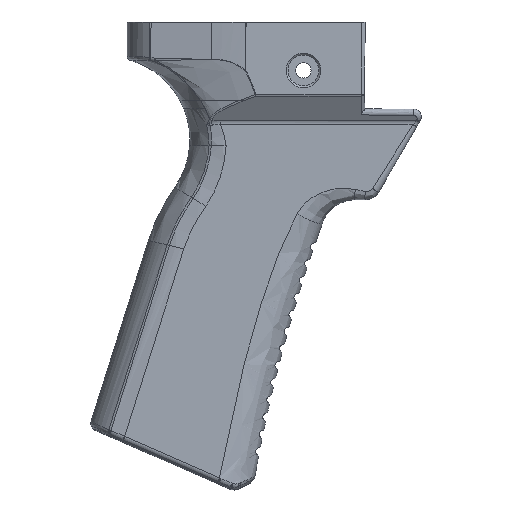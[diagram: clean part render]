
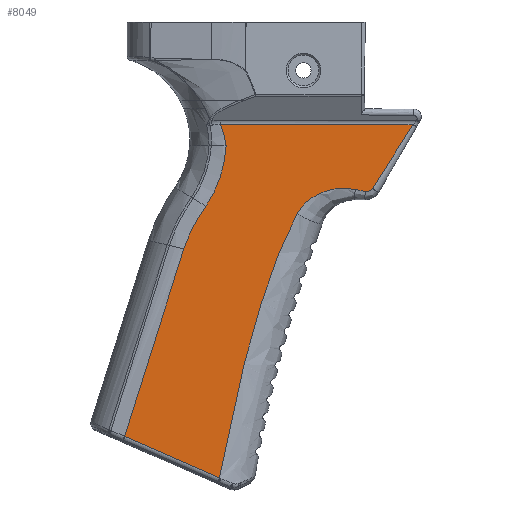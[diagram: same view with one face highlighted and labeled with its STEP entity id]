
A CAD part, front view. The second image highlights one B-rep face of the part: STEP entity #8049.
In plain terms, the highlighted planar face has unit normal (0, -1, 0).
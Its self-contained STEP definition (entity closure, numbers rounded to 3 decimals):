
#165=PLANE('',#8667);
#487=CIRCLE('',#8652,40.554);
#494=CIRCLE('',#8668,30.927);
#1096=FACE_OUTER_BOUND('',#1602,.T.);
#1602=EDGE_LOOP('',(#6779,#6780,#6781,#6782,#6783,#6784,#6785,#6786,#6787,
#6788,#6789,#6790,#6791,#6792));
#1988=LINE('',#18646,#2397);
#1993=LINE('',#19076,#2402);
#2001=LINE('',#19854,#2410);
#2397=VECTOR('',#9956,10.);
#2402=VECTOR('',#9979,10.);
#2410=VECTOR('',#10015,10.);
#2932=B_SPLINE_CURVE_WITH_KNOTS('',3,(#18666,#18667,#18668,#18669),
 .UNSPECIFIED.,.F.,.F.,(4,4),(0.,0.01),.UNSPECIFIED.);
#2937=B_SPLINE_CURVE_WITH_KNOTS('',3,(#18757,#18758,#18759,#18760),
 .UNSPECIFIED.,.F.,.F.,(4,4),(0.,0.007),.UNSPECIFIED.);
#2941=B_SPLINE_CURVE_WITH_KNOTS('',3,(#18888,#18889,#18890,#18891,#18892,
#18893,#18894,#18895,#18896),.UNSPECIFIED.,.F.,.F.,(4,1,1,1,1,1,4),(6.035,
6.926,7.817,9.599,11.381,13.163,
13.222),.UNSPECIFIED.);
#2953=B_SPLINE_CURVE_WITH_KNOTS('',3,(#19226,#19227,#19228,#19229,#19230,
#19231,#19232),.UNSPECIFIED.,.F.,.F.,(4,1,1,1,4),(4.224,5.,
5.518,5.776,5.862),.UNSPECIFIED.);
#2954=B_SPLINE_CURVE_WITH_KNOTS('',3,(#19233,#19234,#19235,#19236),
 .UNSPECIFIED.,.F.,.F.,(4,4),(5.862,6.035),
 .UNSPECIFIED.);
#2956=B_SPLINE_CURVE_WITH_KNOTS('',3,(#19274,#19275,#19276,#19277),
 .UNSPECIFIED.,.F.,.F.,(4,4),(3.956,4.224),
 .UNSPECIFIED.);
#2959=B_SPLINE_CURVE_WITH_KNOTS('',3,(#19326,#19327,#19328,#19329,#19330),
 .UNSPECIFIED.,.F.,.F.,(4,1,4),(3.743,3.835,3.956),
 .UNSPECIFIED.);
#2962=B_SPLINE_CURVE_WITH_KNOTS('',3,(#19380,#19381,#19382,#19383,#19384),
 .UNSPECIFIED.,.F.,.F.,(4,1,4),(1.774,2.899,3.743),
 .UNSPECIFIED.);
#2976=B_SPLINE_CURVE_WITH_KNOTS('',3,(#19856,#19857,#19858,#19859,#19860,
#19861,#19862),.UNSPECIFIED.,.F.,.F.,(4,3,4),(0.258,0.274,
0.412),.UNSPECIFIED.);
#3595=VERTEX_POINT('',#18643);
#3596=VERTEX_POINT('',#18645);
#3597=VERTEX_POINT('',#18664);
#3599=VERTEX_POINT('',#18708);
#3602=VERTEX_POINT('',#18880);
#3608=VERTEX_POINT('',#19011);
#3609=VERTEX_POINT('',#19019);
#3618=VERTEX_POINT('',#19217);
#3619=VERTEX_POINT('',#19225);
#3621=VERTEX_POINT('',#19266);
#3623=VERTEX_POINT('',#19318);
#3625=VERTEX_POINT('',#19372);
#3634=VERTEX_POINT('',#19853);
#3635=VERTEX_POINT('',#19855);
#4657=EDGE_CURVE('',#3595,#3596,#1988,.T.);
#4660=EDGE_CURVE('',#3596,#3597,#2932,.T.);
#4668=EDGE_CURVE('',#3597,#3599,#2937,.T.);
#4672=EDGE_CURVE('',#3602,#3595,#2941,.T.);
#4684=EDGE_CURVE('',#3608,#3609,#487,.T.);
#4687=EDGE_CURVE('',#3609,#3599,#1993,.T.);
#4703=EDGE_CURVE('',#3618,#3619,#2953,.T.);
#4704=EDGE_CURVE('',#3619,#3602,#2954,.T.);
#4706=EDGE_CURVE('',#3621,#3618,#2956,.T.);
#4709=EDGE_CURVE('',#3623,#3621,#2959,.T.);
#4712=EDGE_CURVE('',#3625,#3623,#2962,.T.);
#4728=EDGE_CURVE('',#3634,#3625,#2001,.T.);
#4729=EDGE_CURVE('',#3635,#3634,#2976,.T.);
#4730=EDGE_CURVE('',#3635,#3608,#494,.T.);
#6779=ORIENTED_EDGE('',*,*,#4703,.F.);
#6780=ORIENTED_EDGE('',*,*,#4706,.F.);
#6781=ORIENTED_EDGE('',*,*,#4709,.F.);
#6782=ORIENTED_EDGE('',*,*,#4712,.F.);
#6783=ORIENTED_EDGE('',*,*,#4728,.F.);
#6784=ORIENTED_EDGE('',*,*,#4729,.F.);
#6785=ORIENTED_EDGE('',*,*,#4730,.T.);
#6786=ORIENTED_EDGE('',*,*,#4684,.T.);
#6787=ORIENTED_EDGE('',*,*,#4687,.T.);
#6788=ORIENTED_EDGE('',*,*,#4668,.F.);
#6789=ORIENTED_EDGE('',*,*,#4660,.F.);
#6790=ORIENTED_EDGE('',*,*,#4657,.F.);
#6791=ORIENTED_EDGE('',*,*,#4672,.F.);
#6792=ORIENTED_EDGE('',*,*,#4704,.F.);
#8049=ADVANCED_FACE('',(#1096),#165,.T.);
#8652=AXIS2_PLACEMENT_3D('',#19027,#9975,#9976);
#8667=AXIS2_PLACEMENT_3D('',#19852,#10013,#10014);
#8668=AXIS2_PLACEMENT_3D('',#19863,#10016,#10017);
#9956=DIRECTION('',(-0.916,0.,0.401));
#9975=DIRECTION('center_axis',(0.,-1.,0.));
#9976=DIRECTION('ref_axis',(-0.807,0.,0.591));
#9979=DIRECTION('',(-0.301,0.,-0.953));
#10013=DIRECTION('center_axis',(0.,-1.,0.));
#10014=DIRECTION('ref_axis',(1.,0.,0.));
#10015=DIRECTION('',(1.,0.,-0.002));
#10016=DIRECTION('center_axis',(0.,1.,0.));
#10017=DIRECTION('ref_axis',(0.999,0.,-0.049));
#18643=CARTESIAN_POINT('',(-172.971,4.318,-121.038));
#18645=CARTESIAN_POINT('',(-197.483,4.318,-110.316));
#18646=CARTESIAN_POINT('',(-181.8,4.318,-117.176));
#18664=CARTESIAN_POINT('',(-197.574,4.318,-110.276));
#18666=CARTESIAN_POINT('Ctrl Pts',(-197.483,4.318,-110.316));
#18667=CARTESIAN_POINT('Ctrl Pts',(-197.513,4.318,-110.303));
#18668=CARTESIAN_POINT('Ctrl Pts',(-197.543,4.318,-110.289));
#18669=CARTESIAN_POINT('Ctrl Pts',(-197.574,4.318,-110.276));
#18708=CARTESIAN_POINT('',(-197.637,4.318,-110.248));
#18757=CARTESIAN_POINT('Ctrl Pts',(-197.574,4.318,-110.276));
#18758=CARTESIAN_POINT('Ctrl Pts',(-197.595,4.318,-110.267));
#18759=CARTESIAN_POINT('Ctrl Pts',(-197.616,4.318,-110.257));
#18760=CARTESIAN_POINT('Ctrl Pts',(-197.637,4.318,-110.248));
#18880=CARTESIAN_POINT('',(-152.778,4.318,-52.396));
#18888=CARTESIAN_POINT('Ctrl Pts',(-152.778,4.318,-52.396));
#18889=CARTESIAN_POINT('Ctrl Pts',(-154.228,4.318,-54.941));
#18890=CARTESIAN_POINT('Ctrl Pts',(-156.709,4.318,-60.325));
#18891=CARTESIAN_POINT('Ctrl Pts',(-160.907,4.318,-71.429));
#18892=CARTESIAN_POINT('Ctrl Pts',(-165.172,4.318,-85.667));
#18893=CARTESIAN_POINT('Ctrl Pts',(-169.46,4.318,-102.962));
#18894=CARTESIAN_POINT('Ctrl Pts',(-171.854,4.318,-114.802));
#18895=CARTESIAN_POINT('Ctrl Pts',(-172.936,4.318,-120.844));
#18896=CARTESIAN_POINT('Ctrl Pts',(-172.971,4.318,-121.038));
#19011=CARTESIAN_POINT('',(-176.488,4.318,-50.399));
#19019=CARTESIAN_POINT('',(-182.225,4.318,-61.49));
#19027=CARTESIAN_POINT('Origin',(-143.765,4.318,-74.355));
#19076=CARTESIAN_POINT('',(-182.225,4.318,-61.49));
#19217=CARTESIAN_POINT('',(-137.598,4.318,-46.076));
#19225=CARTESIAN_POINT('',(-151.84,4.318,-50.985));
#19226=CARTESIAN_POINT('Ctrl Pts',(-137.598,4.318,-46.076));
#19227=CARTESIAN_POINT('Ctrl Pts',(-140.069,4.318,-45.535));
#19228=CARTESIAN_POINT('Ctrl Pts',(-144.364,4.318,-45.71));
#19229=CARTESIAN_POINT('Ctrl Pts',(-148.882,4.318,-47.997));
#19230=CARTESIAN_POINT('Ctrl Pts',(-150.951,4.318,-49.894));
#19231=CARTESIAN_POINT('Ctrl Pts',(-151.668,4.318,-50.762));
#19232=CARTESIAN_POINT('Ctrl Pts',(-151.839,4.318,-50.985));
#19233=CARTESIAN_POINT('Ctrl Pts',(-151.839,4.318,-50.985));
#19234=CARTESIAN_POINT('Ctrl Pts',(-152.183,4.318,-51.432));
#19235=CARTESIAN_POINT('Ctrl Pts',(-152.498,4.318,-51.903));
#19236=CARTESIAN_POINT('Ctrl Pts',(-152.778,4.318,-52.396));
#19266=CARTESIAN_POINT('',(-135.016,4.318,-46.573));
#19274=CARTESIAN_POINT('Ctrl Pts',(-135.016,4.318,-46.573));
#19275=CARTESIAN_POINT('Ctrl Pts',(-135.885,4.318,-46.431));
#19276=CARTESIAN_POINT('Ctrl Pts',(-136.746,4.318,-46.263));
#19277=CARTESIAN_POINT('Ctrl Pts',(-137.598,4.318,-46.076));
#19318=CARTESIAN_POINT('',(-133.163,4.318,-45.801));
#19326=CARTESIAN_POINT('Ctrl Pts',(-133.163,4.318,-45.801));
#19327=CARTESIAN_POINT('Ctrl Pts',(-133.345,4.318,-46.042));
#19328=CARTESIAN_POINT('Ctrl Pts',(-133.893,4.318,-46.512));
#19329=CARTESIAN_POINT('Ctrl Pts',(-134.62,4.318,-46.638));
#19330=CARTESIAN_POINT('Ctrl Pts',(-135.016,4.318,-46.573));
#19372=CARTESIAN_POINT('',(-122.649,4.318,-29.188));
#19380=CARTESIAN_POINT('Ctrl Pts',(-122.649,4.318,-29.188));
#19381=CARTESIAN_POINT('Ctrl Pts',(-124.553,4.318,-32.421));
#19382=CARTESIAN_POINT('Ctrl Pts',(-127.885,4.318,-38.078));
#19383=CARTESIAN_POINT('Ctrl Pts',(-131.482,4.318,-43.568));
#19384=CARTESIAN_POINT('Ctrl Pts',(-133.163,4.318,-45.801));
#19852=CARTESIAN_POINT('Origin',(-163.213,4.318,-69.751));
#19853=CARTESIAN_POINT('',(-172.669,4.318,-29.098));
#19854=CARTESIAN_POINT('',(-169.154,4.318,-29.105));
#19855=CARTESIAN_POINT('',(-171.237,4.318,-34.632));
#19856=CARTESIAN_POINT('Ctrl Pts',(-171.237,4.318,-34.632));
#19857=CARTESIAN_POINT('Ctrl Pts',(-171.268,4.318,-34.434));
#19858=CARTESIAN_POINT('Ctrl Pts',(-171.301,4.318,-34.236));
#19859=CARTESIAN_POINT('Ctrl Pts',(-171.337,4.318,-34.039));
#19860=CARTESIAN_POINT('Ctrl Pts',(-171.638,4.318,-32.352));
#19861=CARTESIAN_POINT('Ctrl Pts',(-172.085,4.318,-30.706));
#19862=CARTESIAN_POINT('Ctrl Pts',(-172.669,4.318,-29.098));
#19863=CARTESIAN_POINT('Origin',(-202.126,4.318,-33.103));
